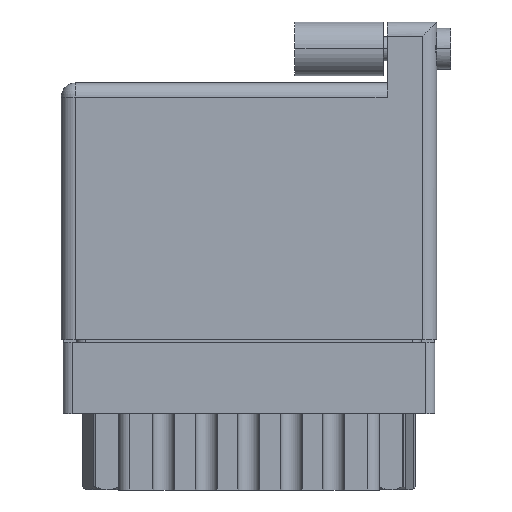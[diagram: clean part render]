
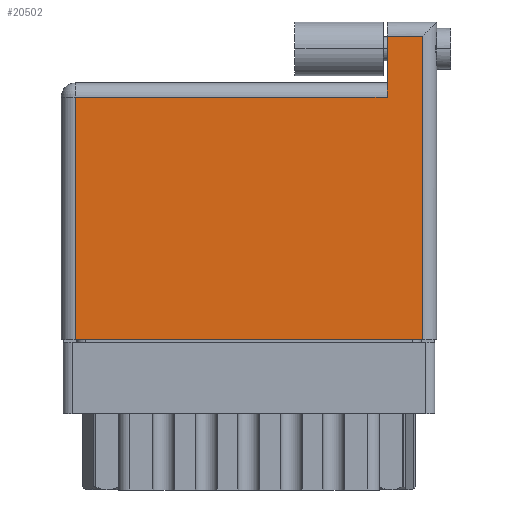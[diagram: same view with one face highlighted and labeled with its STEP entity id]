
A CAD part, front view. The second image highlights one B-rep face of the part: STEP entity #20502.
In plain terms, the highlighted face is planar.
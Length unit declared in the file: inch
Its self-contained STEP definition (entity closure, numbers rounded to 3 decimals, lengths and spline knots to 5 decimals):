
#2 = VECTOR ( 'NONE', #18352, 39.37008 ) ;
#350 = EDGE_CURVE ( 'NONE', #31087, #18630, #38363, .T. ) ;
#996 = VERTEX_POINT ( 'NONE', #8635 ) ;
#1084 = DIRECTION ( 'NONE',  ( 0., -1., 0. ) ) ;
#2640 = EDGE_LOOP ( 'NONE', ( #37557, #38380, #16201, #14728, #9929, #33881 ) ) ;
#2691 = CARTESIAN_POINT ( 'NONE',  ( 1.275, 1.07, 0. ) ) ;
#3811 = EDGE_CURVE ( 'NONE', #4936, #37430, #38220, .T. ) ;
#3827 = DIRECTION ( 'NONE',  ( -1., 0., 0. ) ) ;
#4158 = CARTESIAN_POINT ( 'NONE',  ( 1.275, 1.12, 0. ) ) ;
#4287 = EDGE_CURVE ( 'NONE', #18630, #35203, #36295, .T. ) ;
#4542 = DIRECTION ( 'NONE',  ( -1., 0., 0. ) ) ;
#4936 = VERTEX_POINT ( 'NONE', #29343 ) ;
#5802 = PLANE ( 'NONE',  #6893 ) ;
#6893 = AXIS2_PLACEMENT_3D ( 'NONE', #35738, #38756, #26720 ) ;
#7347 = CARTESIAN_POINT ( 'NONE',  ( 0.05, 0., 0. ) ) ;
#8093 = LINE ( 'NONE', #36013, #2 ) ;
#8635 = CARTESIAN_POINT ( 'NONE',  ( 1.15, 0.856, 0. ) ) ;
#9326 = VECTOR ( 'NONE', #4542, 39.37008 ) ;
#9929 = ORIENTED_EDGE ( 'NONE', *, *, #19805, .T. ) ;
#11647 = FACE_OUTER_BOUND ( 'NONE', #2640, .T. ) ;
#12520 = CARTESIAN_POINT ( 'NONE',  ( 0., 1.07, 0. ) ) ;
#12834 = EDGE_CURVE ( 'NONE', #35203, #996, #8093, .T. ) ;
#13504 = DIRECTION ( 'NONE',  ( 0., 1., 0. ) ) ;
#14378 = CARTESIAN_POINT ( 'NONE',  ( 1.15, 1.07, 0. ) ) ;
#14728 = ORIENTED_EDGE ( 'NONE', *, *, #12834, .T. ) ;
#16201 = ORIENTED_EDGE ( 'NONE', *, *, #4287, .T. ) ;
#16884 = DIRECTION ( 'NONE',  ( 1., 0., 0. ) ) ;
#18352 = DIRECTION ( 'NONE',  ( 0., -1., 0. ) ) ;
#18630 = VERTEX_POINT ( 'NONE', #2691 ) ;
#19239 = VECTOR ( 'NONE', #1084, 39.37008 ) ;
#19805 = EDGE_CURVE ( 'NONE', #996, #4936, #22679, .T. ) ;
#20419 = EDGE_CURVE ( 'NONE', #37430, #31087, #26452, .T. ) ;
#20501 = CARTESIAN_POINT ( 'NONE',  ( 1.275, 0., 0. ) ) ;
#20502 = ADVANCED_FACE ( 'NONE', ( #11647 ), #5802, .F. ) ;
#22679 = LINE ( 'NONE', #22811, #9326 ) ;
#22811 = CARTESIAN_POINT ( 'NONE',  ( 0., 0.856, 0. ) ) ;
#25103 = VECTOR ( 'NONE', #13504, 39.37008 ) ;
#26452 = LINE ( 'NONE', #32024, #33559 ) ;
#26720 = DIRECTION ( 'NONE',  ( -1., 0., 0. ) ) ;
#28513 = CARTESIAN_POINT ( 'NONE',  ( 0.05, 0., 0. ) ) ;
#29343 = CARTESIAN_POINT ( 'NONE',  ( 0.05, 0.856, 0. ) ) ;
#31087 = VERTEX_POINT ( 'NONE', #20501 ) ;
#32024 = CARTESIAN_POINT ( 'NONE',  ( 0., 0., 0. ) ) ;
#33559 = VECTOR ( 'NONE', #16884, 39.37008 ) ;
#33881 = ORIENTED_EDGE ( 'NONE', *, *, #3811, .T. ) ;
#33933 = VECTOR ( 'NONE', #3827, 39.37008 ) ;
#35203 = VERTEX_POINT ( 'NONE', #14378 ) ;
#35738 = CARTESIAN_POINT ( 'NONE',  ( 0., 0.906, 0. ) ) ;
#36013 = CARTESIAN_POINT ( 'NONE',  ( 1.15, 1.12, 0. ) ) ;
#36295 = LINE ( 'NONE', #12520, #33933 ) ;
#37430 = VERTEX_POINT ( 'NONE', #7347 ) ;
#37557 = ORIENTED_EDGE ( 'NONE', *, *, #20419, .T. ) ;
#38220 = LINE ( 'NONE', #28513, #19239 ) ;
#38363 = LINE ( 'NONE', #4158, #25103 ) ;
#38380 = ORIENTED_EDGE ( 'NONE', *, *, #350, .T. ) ;
#38756 = DIRECTION ( 'NONE',  ( 0., 0., -1. ) ) ;
